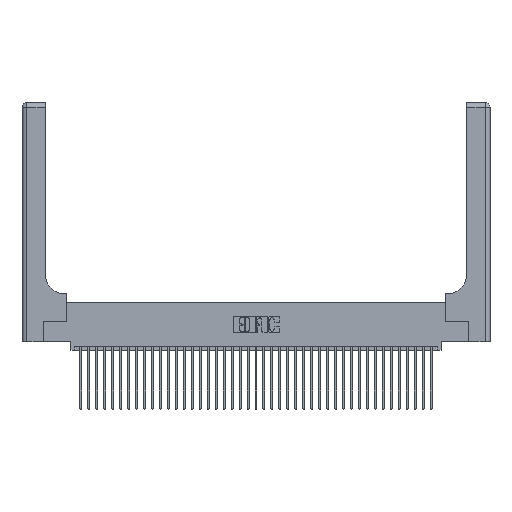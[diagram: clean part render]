
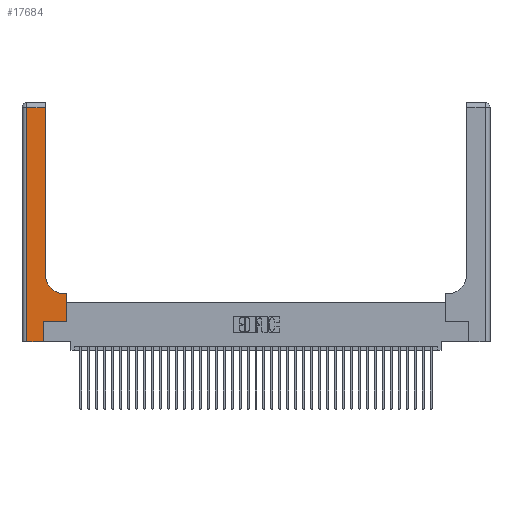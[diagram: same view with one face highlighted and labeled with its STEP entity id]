
A CAD part, top view. The second image highlights one B-rep face of the part: STEP entity #17684.
In plain terms, the highlighted planar face has unit normal (0, 0, 1).
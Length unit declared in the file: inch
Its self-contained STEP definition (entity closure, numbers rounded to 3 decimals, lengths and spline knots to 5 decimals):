
#300 = LINE ( 'NONE', #31833, #24217 ) ;
#477 = CARTESIAN_POINT ( 'NONE',  ( 0.269, 0.25, 0.37 ) ) ;
#879 = VECTOR ( 'NONE', #27342, 39.37008 ) ;
#1311 = VECTOR ( 'NONE', #26842, 39.37008 ) ;
#1592 = CARTESIAN_POINT ( 'NONE',  ( 0.5585, 0.25, 0.37 ) ) ;
#2449 = EDGE_CURVE ( 'NONE', #9312, #31043, #6993, .T. ) ;
#2597 = DIRECTION ( 'NONE',  ( -1., 0., 0. ) ) ;
#3987 = VECTOR ( 'NONE', #13374, 39.37008 ) ;
#5033 = CARTESIAN_POINT ( 'NONE',  ( 0., 2.94, 0.37 ) ) ;
#5197 = VECTOR ( 'NONE', #10201, 39.37008 ) ;
#5390 = CARTESIAN_POINT ( 'NONE',  ( 0.5415, 0.6, 0.37 ) ) ;
#6380 = EDGE_CURVE ( 'NONE', #11921, #19117, #16913, .T. ) ;
#6993 = CIRCLE ( 'NONE', #24256, 0.25 ) ;
#7146 = EDGE_CURVE ( 'NONE', #28509, #21103, #25765, .T. ) ;
#7752 = ORIENTED_EDGE ( 'NONE', *, *, #20520, .T. ) ;
#9312 = VERTEX_POINT ( 'NONE', #5390 ) ;
#10201 = DIRECTION ( 'NONE',  ( 1., 0., 0. ) ) ;
#10623 = FACE_OUTER_BOUND ( 'NONE', #20686, .T. ) ;
#11035 = EDGE_CURVE ( 'NONE', #23366, #9312, #21113, .T. ) ;
#11110 = CARTESIAN_POINT ( 'NONE',  ( 0.269, 0., 0.37 ) ) ;
#11921 = VERTEX_POINT ( 'NONE', #34513 ) ;
#12477 = ORIENTED_EDGE ( 'NONE', *, *, #17952, .T. ) ;
#12493 = LINE ( 'NONE', #28875, #5197 ) ;
#13374 = DIRECTION ( 'NONE',  ( 0., -1., 0. ) ) ;
#13962 = DIRECTION ( 'NONE',  ( 0., 0., -1. ) ) ;
#14199 = ORIENTED_EDGE ( 'NONE', *, *, #33918, .T. ) ;
#15713 = CARTESIAN_POINT ( 'NONE',  ( 0.06, 0., 0.37 ) ) ;
#16319 = DIRECTION ( 'NONE',  ( 0., 1., 0. ) ) ;
#16791 = CARTESIAN_POINT ( 'NONE',  ( 0.2915, 0.85, 0.37 ) ) ;
#16913 = LINE ( 'NONE', #5033, #1311 ) ;
#17445 = VECTOR ( 'NONE', #22373, 39.37008 ) ;
#17684 = ADVANCED_FACE ( 'NONE', ( #10623 ), #36607, .F. ) ;
#17857 = CARTESIAN_POINT ( 'NONE',  ( 0.269, 0.25, 0.37 ) ) ;
#17952 = EDGE_CURVE ( 'NONE', #31043, #11921, #33984, .T. ) ;
#18044 = DIRECTION ( 'NONE',  ( 0., 0., -1. ) ) ;
#18686 = EDGE_CURVE ( 'NONE', #29866, #23366, #300, .T. ) ;
#19117 = VERTEX_POINT ( 'NONE', #33717 ) ;
#19243 = CARTESIAN_POINT ( 'NONE',  ( 0.2915, 3., 0.37 ) ) ;
#20286 = CARTESIAN_POINT ( 'NONE',  ( 0.5585, 0.6, 0.37 ) ) ;
#20520 = EDGE_CURVE ( 'NONE', #22503, #28509, #12493, .T. ) ;
#20686 = EDGE_LOOP ( 'NONE', ( #12477, #25950, #21649, #7752, #26902, #14199, #22028, #34459, #38206 ) ) ;
#21103 = VERTEX_POINT ( 'NONE', #477 ) ;
#21113 = LINE ( 'NONE', #39819, #36626 ) ;
#21649 = ORIENTED_EDGE ( 'NONE', *, *, #29016, .T. ) ;
#22028 = ORIENTED_EDGE ( 'NONE', *, *, #18686, .T. ) ;
#22373 = DIRECTION ( 'NONE',  ( 0., 1., 0. ) ) ;
#22503 = VERTEX_POINT ( 'NONE', #15713 ) ;
#22752 = AXIS2_PLACEMENT_3D ( 'NONE', #30426, #18044, #39714 ) ;
#23366 = VERTEX_POINT ( 'NONE', #20286 ) ;
#24217 = VECTOR ( 'NONE', #16319, 39.37008 ) ;
#24256 = AXIS2_PLACEMENT_3D ( 'NONE', #32590, #13962, #35673 ) ;
#25765 = LINE ( 'NONE', #30457, #879 ) ;
#25950 = ORIENTED_EDGE ( 'NONE', *, *, #6380, .T. ) ;
#26842 = DIRECTION ( 'NONE',  ( -1., 0., 0. ) ) ;
#26902 = ORIENTED_EDGE ( 'NONE', *, *, #7146, .T. ) ;
#27265 = DIRECTION ( 'NONE',  ( 1., 0., 0. ) ) ;
#27342 = DIRECTION ( 'NONE',  ( 0., 1., 0. ) ) ;
#28509 = VERTEX_POINT ( 'NONE', #11110 ) ;
#28860 = LINE ( 'NONE', #28910, #3987 ) ;
#28875 = CARTESIAN_POINT ( 'NONE',  ( 0., 0., 0.37 ) ) ;
#28910 = CARTESIAN_POINT ( 'NONE',  ( 0.06, 3., 0.37 ) ) ;
#29016 = EDGE_CURVE ( 'NONE', #19117, #22503, #28860, .T. ) ;
#29019 = VECTOR ( 'NONE', #27265, 39.37008 ) ;
#29866 = VERTEX_POINT ( 'NONE', #1592 ) ;
#30011 = LINE ( 'NONE', #17857, #29019 ) ;
#30426 = CARTESIAN_POINT ( 'NONE',  ( 0., 3., 0.37 ) ) ;
#30457 = CARTESIAN_POINT ( 'NONE',  ( 0.269, 0., 0.37 ) ) ;
#31043 = VERTEX_POINT ( 'NONE', #16791 ) ;
#31833 = CARTESIAN_POINT ( 'NONE',  ( 0.5585, 0.25, 0.37 ) ) ;
#32590 = CARTESIAN_POINT ( 'NONE',  ( 0.5415, 0.85, 0.37 ) ) ;
#33717 = CARTESIAN_POINT ( 'NONE',  ( 0.06, 2.94, 0.37 ) ) ;
#33918 = EDGE_CURVE ( 'NONE', #21103, #29866, #30011, .T. ) ;
#33984 = LINE ( 'NONE', #19243, #17445 ) ;
#34459 = ORIENTED_EDGE ( 'NONE', *, *, #11035, .T. ) ;
#34513 = CARTESIAN_POINT ( 'NONE',  ( 0.2915, 2.94, 0.37 ) ) ;
#35673 = DIRECTION ( 'NONE',  ( 1., 0., 0. ) ) ;
#36607 = PLANE ( 'NONE',  #22752 ) ;
#36626 = VECTOR ( 'NONE', #2597, 39.37008 ) ;
#38206 = ORIENTED_EDGE ( 'NONE', *, *, #2449, .T. ) ;
#39714 = DIRECTION ( 'NONE',  ( -1., 0., 0. ) ) ;
#39819 = CARTESIAN_POINT ( 'NONE',  ( 0.2915, 0.6, 0.37 ) ) ;
